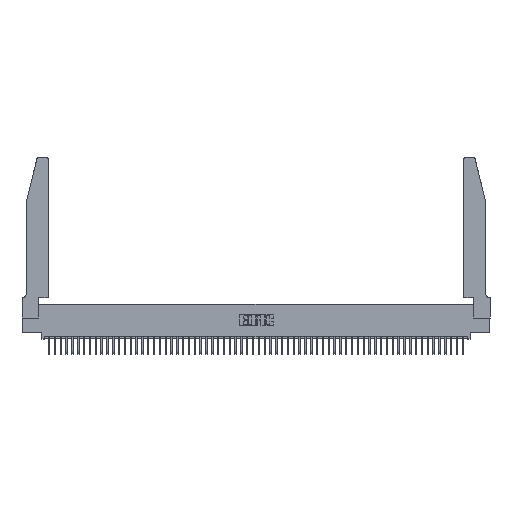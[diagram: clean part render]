
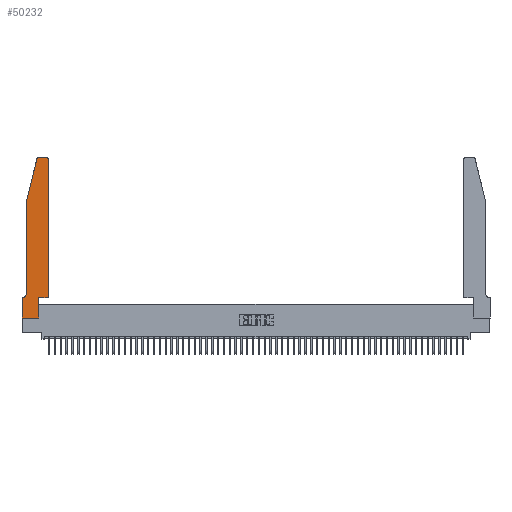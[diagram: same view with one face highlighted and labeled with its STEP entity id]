
A CAD part, top view. The second image highlights one B-rep face of the part: STEP entity #50232.
In plain terms, the highlighted planar face has unit normal (0, 0, 1).
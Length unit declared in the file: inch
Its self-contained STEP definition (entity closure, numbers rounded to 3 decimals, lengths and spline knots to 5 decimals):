
#87 = CARTESIAN_POINT ( 'NONE',  ( 0.284, 2.75, 0.37 ) ) ;
#309 = LINE ( 'NONE', #9259, #1653 ) ;
#875 = VECTOR ( 'NONE', #8597, 39.37008 ) ;
#1222 = CARTESIAN_POINT ( 'NONE',  ( 0.2865, 0.35, 0.37 ) ) ;
#1653 = VECTOR ( 'NONE', #39000, 39.37008 ) ;
#2628 = DIRECTION ( 'NONE',  ( 1., 0., 0. ) ) ;
#2872 = CARTESIAN_POINT ( 'NONE',  ( 0.4505, 2.72, 0.37 ) ) ;
#3016 = ORIENTED_EDGE ( 'NONE', *, *, #23959, .T. ) ;
#3588 = EDGE_CURVE ( 'NONE', #39205, #18270, #6840, .T. ) ;
#4006 = DIRECTION ( 'NONE',  ( 1., 0., 0. ) ) ;
#4793 = VECTOR ( 'NONE', #9257, 39.37008 ) ;
#5277 = AXIS2_PLACEMENT_3D ( 'NONE', #45025, #28192, #2628 ) ;
#5348 = CARTESIAN_POINT ( 'NONE',  ( 0.0055, 0.42, 0.37 ) ) ;
#6044 = DIRECTION ( 'NONE',  ( 0., -1., 0. ) ) ;
#6466 = CARTESIAN_POINT ( 'NONE',  ( 0.2865, 0., 0.37 ) ) ;
#6630 = CARTESIAN_POINT ( 'NONE',  ( 0.0755, 0.42, 0.37 ) ) ;
#6840 = LINE ( 'NONE', #48329, #16874 ) ;
#6876 = EDGE_CURVE ( 'NONE', #42830, #36685, #27145, .T. ) ;
#8597 = DIRECTION ( 'NONE',  ( -1., 0., 0. ) ) ;
#9257 = DIRECTION ( 'NONE',  ( -0.239, -0.971, 0. ) ) ;
#9259 = CARTESIAN_POINT ( 'NONE',  ( 0.4505, 0.35, 0.37 ) ) ;
#9639 = DIRECTION ( 'NONE',  ( -1., 0., 0. ) ) ;
#9908 = DIRECTION ( 'NONE',  ( 0., -1., 0. ) ) ;
#10183 = VERTEX_POINT ( 'NONE', #17163 ) ;
#10235 = DIRECTION ( 'NONE',  ( 0., 1., 0. ) ) ;
#11403 = CARTESIAN_POINT ( 'NONE',  ( 0.0755, 2., 0.37 ) ) ;
#11420 = VECTOR ( 'NONE', #9908, 39.37008 ) ;
#12202 = ORIENTED_EDGE ( 'NONE', *, *, #38547, .T. ) ;
#12266 = LINE ( 'NONE', #29858, #875 ) ;
#13479 = LINE ( 'NONE', #48130, #34767 ) ;
#14474 = CIRCLE ( 'NONE', #35200, 0.03 ) ;
#16440 = ORIENTED_EDGE ( 'NONE', *, *, #6876, .T. ) ;
#16464 = VERTEX_POINT ( 'NONE', #44989 ) ;
#16874 = VECTOR ( 'NONE', #10235, 39.37008 ) ;
#17002 = CARTESIAN_POINT ( 'NONE',  ( 0.4205, 2.72, 0.37 ) ) ;
#17163 = CARTESIAN_POINT ( 'NONE',  ( 0., 0., 0.37 ) ) ;
#17697 = AXIS2_PLACEMENT_3D ( 'NONE', #17002, #46687, #21329 ) ;
#17846 = CARTESIAN_POINT ( 'NONE',  ( 0.0755, 2., 0.37 ) ) ;
#18050 = CARTESIAN_POINT ( 'NONE',  ( 0.4505, 0.35, 0.37 ) ) ;
#18270 = VERTEX_POINT ( 'NONE', #1222 ) ;
#19045 = LINE ( 'NONE', #25130, #51571 ) ;
#20702 = EDGE_CURVE ( 'NONE', #10183, #39205, #19045, .T. ) ;
#20747 = CARTESIAN_POINT ( 'NONE',  ( 0.2605, 2.75, 0.37 ) ) ;
#21329 = DIRECTION ( 'NONE',  ( 1., 0., 0. ) ) ;
#21812 = CARTESIAN_POINT ( 'NONE',  ( 0.0055, 0.35, 0.37 ) ) ;
#22207 = ORIENTED_EDGE ( 'NONE', *, *, #35777, .T. ) ;
#22612 = VERTEX_POINT ( 'NONE', #87 ) ;
#23679 = FACE_OUTER_BOUND ( 'NONE', #27120, .T. ) ;
#23959 = EDGE_CURVE ( 'NONE', #18270, #33844, #13479, .T. ) ;
#24715 = VECTOR ( 'NONE', #25002, 39.37008 ) ;
#25002 = DIRECTION ( 'NONE',  ( -1., 0., 0. ) ) ;
#25130 = CARTESIAN_POINT ( 'NONE',  ( 0., 0., 0.37 ) ) ;
#25560 = EDGE_CURVE ( 'NONE', #37330, #22612, #34678, .T. ) ;
#26519 = ORIENTED_EDGE ( 'NONE', *, *, #49093, .T. ) ;
#27120 = EDGE_LOOP ( 'NONE', ( #54971, #26519, #40234, #16440, #38286, #34415, #12202, #40975, #36340, #3016, #27441, #22207 ) ) ;
#27145 = LINE ( 'NONE', #35821, #48348 ) ;
#27441 = ORIENTED_EDGE ( 'NONE', *, *, #41774, .T. ) ;
#28192 = DIRECTION ( 'NONE',  ( 0., 0., 1. ) ) ;
#29569 = DIRECTION ( 'NONE',  ( 0., 0., 1. ) ) ;
#29858 = CARTESIAN_POINT ( 'NONE',  ( 0.0755, 0.35, 0.37 ) ) ;
#31352 = VERTEX_POINT ( 'NONE', #49122 ) ;
#32839 = CARTESIAN_POINT ( 'NONE',  ( 0.4205, 2.75, 0.37 ) ) ;
#33844 = VERTEX_POINT ( 'NONE', #18050 ) ;
#34415 = ORIENTED_EDGE ( 'NONE', *, *, #44539, .T. ) ;
#34678 = LINE ( 'NONE', #20747, #24715 ) ;
#34767 = VECTOR ( 'NONE', #39592, 39.37008 ) ;
#35138 = DIRECTION ( 'NONE',  ( 0., 0., -1. ) ) ;
#35200 = AXIS2_PLACEMENT_3D ( 'NONE', #54918, #29569, #4006 ) ;
#35383 = CARTESIAN_POINT ( 'NONE',  ( 0., 0., 0.37 ) ) ;
#35508 = AXIS2_PLACEMENT_3D ( 'NONE', #5348, #35138, #9639 ) ;
#35777 = EDGE_CURVE ( 'NONE', #45673, #37330, #40334, .T. ) ;
#35821 = CARTESIAN_POINT ( 'NONE',  ( 0.0755, 2., 0.37 ) ) ;
#36340 = ORIENTED_EDGE ( 'NONE', *, *, #3588, .T. ) ;
#36502 = EDGE_CURVE ( 'NONE', #36685, #46797, #36932, .T. ) ;
#36685 = VERTEX_POINT ( 'NONE', #6630 ) ;
#36932 = CIRCLE ( 'NONE', #35508, 0.07 ) ;
#37330 = VERTEX_POINT ( 'NONE', #32839 ) ;
#38286 = ORIENTED_EDGE ( 'NONE', *, *, #36502, .T. ) ;
#38547 = EDGE_CURVE ( 'NONE', #31352, #10183, #42641, .T. ) ;
#39000 = DIRECTION ( 'NONE',  ( 0., 1., 0. ) ) ;
#39205 = VERTEX_POINT ( 'NONE', #6466 ) ;
#39592 = DIRECTION ( 'NONE',  ( 1., 0., 0. ) ) ;
#40234 = ORIENTED_EDGE ( 'NONE', *, *, #45311, .T. ) ;
#40334 = CIRCLE ( 'NONE', #17697, 0.03 ) ;
#40975 = ORIENTED_EDGE ( 'NONE', *, *, #20702, .T. ) ;
#41774 = EDGE_CURVE ( 'NONE', #33844, #45673, #309, .T. ) ;
#42641 = LINE ( 'NONE', #35383, #11420 ) ;
#42830 = VERTEX_POINT ( 'NONE', #11403 ) ;
#44539 = EDGE_CURVE ( 'NONE', #46797, #31352, #12266, .T. ) ;
#44989 = CARTESIAN_POINT ( 'NONE',  ( 0.25487, 2.72718, 0.37 ) ) ;
#45025 = CARTESIAN_POINT ( 'NONE',  ( 0., 0.35, 0.37 ) ) ;
#45311 = EDGE_CURVE ( 'NONE', #16464, #42830, #48700, .T. ) ;
#45673 = VERTEX_POINT ( 'NONE', #2872 ) ;
#46687 = DIRECTION ( 'NONE',  ( 0., 0., 1. ) ) ;
#46797 = VERTEX_POINT ( 'NONE', #21812 ) ;
#48130 = CARTESIAN_POINT ( 'NONE',  ( 0.4505, 0.35, 0.37 ) ) ;
#48329 = CARTESIAN_POINT ( 'NONE',  ( 0.2865, 0.35, 0.37 ) ) ;
#48348 = VECTOR ( 'NONE', #6044, 39.37008 ) ;
#48700 = LINE ( 'NONE', #17846, #4793 ) ;
#49093 = EDGE_CURVE ( 'NONE', #22612, #16464, #14474, .T. ) ;
#49122 = CARTESIAN_POINT ( 'NONE',  ( 0., 0.35, 0.37 ) ) ;
#50232 = ADVANCED_FACE ( 'NONE', ( #23679 ), #53545, .T. ) ;
#50490 = DIRECTION ( 'NONE',  ( 1., 0., 0. ) ) ;
#51571 = VECTOR ( 'NONE', #50490, 39.37008 ) ;
#53545 = PLANE ( 'NONE',  #5277 ) ;
#54918 = CARTESIAN_POINT ( 'NONE',  ( 0.284, 2.72, 0.37 ) ) ;
#54971 = ORIENTED_EDGE ( 'NONE', *, *, #25560, .T. ) ;
